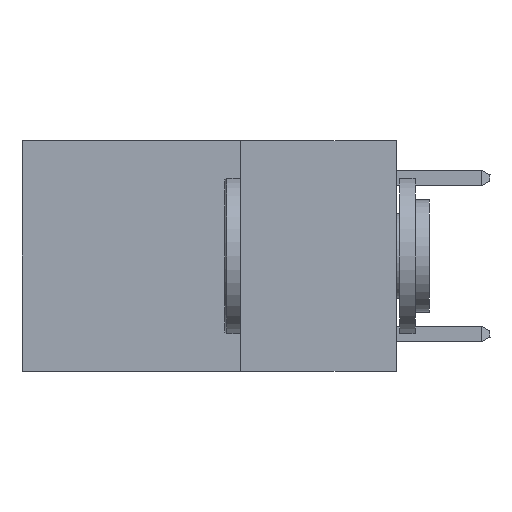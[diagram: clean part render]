
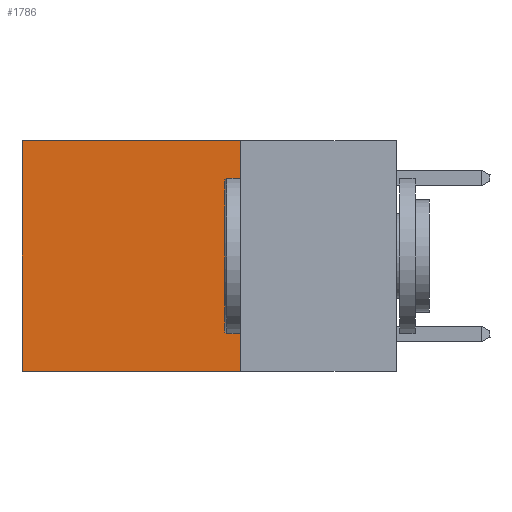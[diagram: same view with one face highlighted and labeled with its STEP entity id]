
A CAD part, left-side view. The second image highlights one B-rep face of the part: STEP entity #1786.
In plain terms, the highlighted planar face has unit normal (-1, 0, 0).
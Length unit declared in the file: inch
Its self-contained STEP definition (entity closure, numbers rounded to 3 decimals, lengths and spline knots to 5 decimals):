
#540 = CARTESIAN_POINT ( 'NONE',  ( 0.2625, 0.6, 0. ) ) ;
#796 = DIRECTION ( 'NONE',  ( 0., 0., -1. ) ) ;
#1317 = CARTESIAN_POINT ( 'NONE',  ( 0.2625, 0.25, 0. ) ) ;
#1786 = ADVANCED_FACE ( 'NONE', ( #14058 ), #14293, .F. ) ;
#4080 = VECTOR ( 'NONE', #4160, 39.37008 ) ;
#4160 = DIRECTION ( 'NONE',  ( 0., 0., -1. ) ) ;
#4718 = LINE ( 'NONE', #6158, #16815 ) ;
#5571 = EDGE_CURVE ( 'NONE', #15148, #13095, #4718, .T. ) ;
#6158 = CARTESIAN_POINT ( 'NONE',  ( 0.2625, 0.25, 0. ) ) ;
#6718 = DIRECTION ( 'NONE',  ( 0., 1., 0. ) ) ;
#7134 = EDGE_CURVE ( 'NONE', #13095, #13830, #19223, .T. ) ;
#7332 = CARTESIAN_POINT ( 'NONE',  ( 0.2625, 0.25, 0. ) ) ;
#8484 = VECTOR ( 'NONE', #21409, 39.37008 ) ;
#8496 = CARTESIAN_POINT ( 'NONE',  ( 0.2625, 0.25, -0.37 ) ) ;
#10007 = AXIS2_PLACEMENT_3D ( 'NONE', #7332, #15946, #796 ) ;
#11504 = DIRECTION ( 'NONE',  ( 0., 1., 0. ) ) ;
#12255 = VERTEX_POINT ( 'NONE', #15748 ) ;
#12828 = LINE ( 'NONE', #1317, #8484 ) ;
#13095 = VERTEX_POINT ( 'NONE', #540 ) ;
#13733 = CARTESIAN_POINT ( 'NONE',  ( 0.2625, 0.6, -0.37 ) ) ;
#13830 = VERTEX_POINT ( 'NONE', #13733 ) ;
#14058 = FACE_OUTER_BOUND ( 'NONE', #17666, .T. ) ;
#14293 = PLANE ( 'NONE',  #10007 ) ;
#14499 = EDGE_CURVE ( 'NONE', #15148, #12255, #12828, .T. ) ;
#15129 = CARTESIAN_POINT ( 'NONE',  ( 0.2625, 0.25, 0. ) ) ;
#15148 = VERTEX_POINT ( 'NONE', #15129 ) ;
#15149 = ORIENTED_EDGE ( 'NONE', *, *, #7134, .T. ) ;
#15199 = ORIENTED_EDGE ( 'NONE', *, *, #5571, .T. ) ;
#15748 = CARTESIAN_POINT ( 'NONE',  ( 0.2625, 0.25, -0.37 ) ) ;
#15946 = DIRECTION ( 'NONE',  ( 1., 0., 0. ) ) ;
#16278 = ORIENTED_EDGE ( 'NONE', *, *, #14499, .F. ) ;
#16815 = VECTOR ( 'NONE', #11504, 39.37008 ) ;
#16875 = LINE ( 'NONE', #8496, #20173 ) ;
#17666 = EDGE_LOOP ( 'NONE', ( #15149, #20162, #16278, #15199 ) ) ;
#18386 = EDGE_CURVE ( 'NONE', #12255, #13830, #16875, .T. ) ;
#19223 = LINE ( 'NONE', #19438, #4080 ) ;
#19438 = CARTESIAN_POINT ( 'NONE',  ( 0.2625, 0.6, 0. ) ) ;
#20162 = ORIENTED_EDGE ( 'NONE', *, *, #18386, .F. ) ;
#20173 = VECTOR ( 'NONE', #6718, 39.37008 ) ;
#21409 = DIRECTION ( 'NONE',  ( 0., 0., -1. ) ) ;
